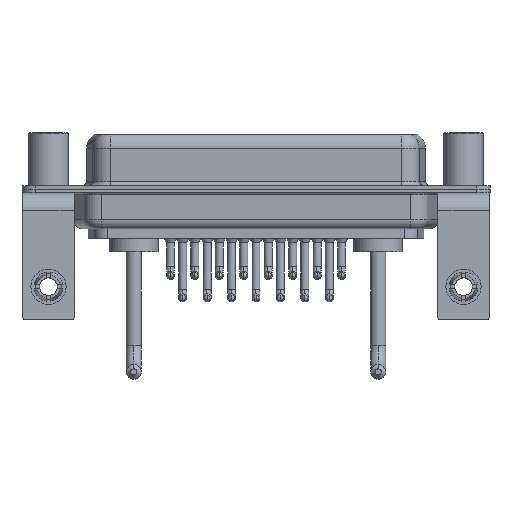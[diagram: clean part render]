
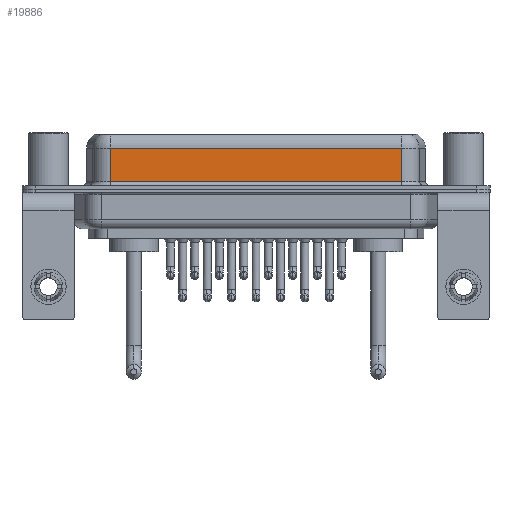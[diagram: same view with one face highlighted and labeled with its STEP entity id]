
A CAD part, front view. The second image highlights one B-rep face of the part: STEP entity #19886.
In plain terms, the highlighted planar face has unit normal (0, -1, 0).
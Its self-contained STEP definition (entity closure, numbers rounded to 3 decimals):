
#458 = ORIENTED_EDGE ( 'NONE', *, *, #11633, .T. ) ;
#1679 = CARTESIAN_POINT ( 'NONE',  ( 40.037, -3.95, 0.9 ) ) ;
#1998 = AXIS2_PLACEMENT_3D ( 'NONE', #13650, #19296, #5972 ) ;
#2132 = VERTEX_POINT ( 'NONE', #2575 ) ;
#2460 = CARTESIAN_POINT ( 'NONE',  ( 40.037, -3.95, 4.65 ) ) ;
#2575 = CARTESIAN_POINT ( 'NONE',  ( 7.013, -3.95, 4.65 ) ) ;
#3665 = EDGE_CURVE ( 'NONE', #2132, #15164, #6576, .T. ) ;
#3989 = FACE_OUTER_BOUND ( 'NONE', #6058, .T. ) ;
#4470 = VECTOR ( 'NONE', #13351, 1000. ) ;
#4593 = CARTESIAN_POINT ( 'NONE',  ( 7.013, -3.95, 6.4 ) ) ;
#4695 = CARTESIAN_POINT ( 'NONE',  ( 40.037, -3.95, 6.4 ) ) ;
#5474 = CARTESIAN_POINT ( 'NONE',  ( 40.037, -3.95, 4.65 ) ) ;
#5551 = EDGE_CURVE ( 'NONE', #24082, #12407, #21616, .T. ) ;
#5972 = DIRECTION ( 'NONE',  ( 0., 0., 1. ) ) ;
#6058 = EDGE_LOOP ( 'NONE', ( #17935, #458, #11685, #11967 ) ) ;
#6576 = LINE ( 'NONE', #4593, #11281 ) ;
#6993 = DIRECTION ( 'NONE',  ( 1., 0., 0. ) ) ;
#10404 = DIRECTION ( 'NONE',  ( 0., 0., -1. ) ) ;
#10430 = DIRECTION ( 'NONE',  ( 0., 0., -1. ) ) ;
#10960 = LINE ( 'NONE', #1679, #16327 ) ;
#11281 = VECTOR ( 'NONE', #10430, 1000. ) ;
#11552 = PLANE ( 'NONE',  #1998 ) ;
#11633 = EDGE_CURVE ( 'NONE', #24082, #2132, #11994, .T. ) ;
#11685 = ORIENTED_EDGE ( 'NONE', *, *, #3665, .T. ) ;
#11967 = ORIENTED_EDGE ( 'NONE', *, *, #13768, .T. ) ;
#11994 = LINE ( 'NONE', #2460, #4470 ) ;
#12407 = VERTEX_POINT ( 'NONE', #18241 ) ;
#13351 = DIRECTION ( 'NONE',  ( -1., 0., 0. ) ) ;
#13650 = CARTESIAN_POINT ( 'NONE',  ( 40.037, -3.95, 6.4 ) ) ;
#13768 = EDGE_CURVE ( 'NONE', #15164, #12407, #10960, .T. ) ;
#15164 = VERTEX_POINT ( 'NONE', #15726 ) ;
#15726 = CARTESIAN_POINT ( 'NONE',  ( 7.013, -3.95, 0.9 ) ) ;
#16327 = VECTOR ( 'NONE', #6993, 1000. ) ;
#17935 = ORIENTED_EDGE ( 'NONE', *, *, #5551, .F. ) ;
#18241 = CARTESIAN_POINT ( 'NONE',  ( 40.037, -3.95, 0.9 ) ) ;
#19296 = DIRECTION ( 'NONE',  ( 0., 1., 0. ) ) ;
#19886 = ADVANCED_FACE ( 'NONE', ( #3989 ), #11552, .F. ) ;
#20005 = VECTOR ( 'NONE', #10404, 1000. ) ;
#21616 = LINE ( 'NONE', #4695, #20005 ) ;
#24082 = VERTEX_POINT ( 'NONE', #5474 ) ;
